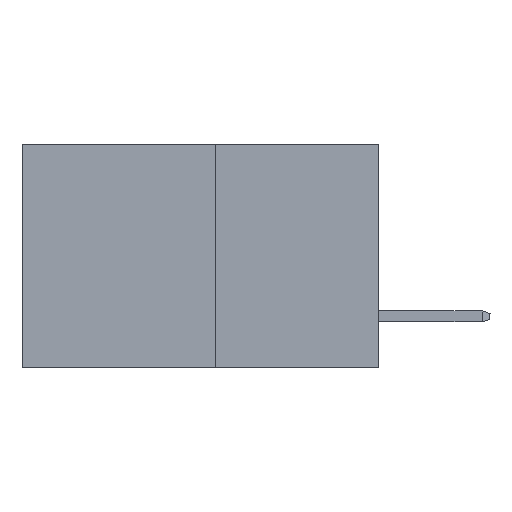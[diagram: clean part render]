
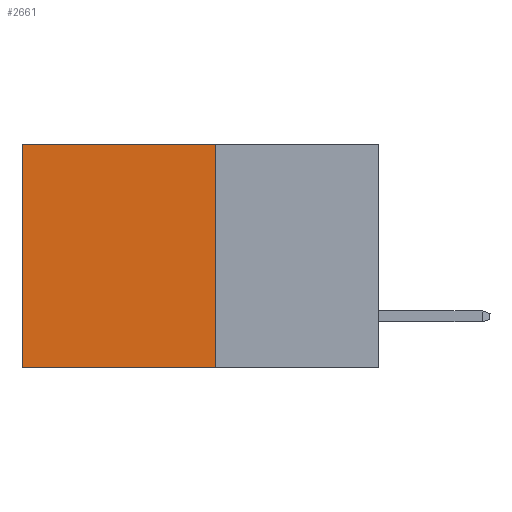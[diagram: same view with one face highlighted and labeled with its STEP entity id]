
A CAD part, left-side view. The second image highlights one B-rep face of the part: STEP entity #2661.
In plain terms, the highlighted planar face has unit normal (-1, 0, 0).
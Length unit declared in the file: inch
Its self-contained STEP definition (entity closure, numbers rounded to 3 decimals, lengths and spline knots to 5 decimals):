
#350 = LINE ( 'NONE', #3669, #9872 ) ;
#476 = EDGE_CURVE ( 'NONE', #3272, #10678, #350, .T. ) ;
#968 = EDGE_CURVE ( 'NONE', #11076, #4320, #6662, .T. ) ;
#1691 = VECTOR ( 'NONE', #6473, 39.37008 ) ;
#2283 = ORIENTED_EDGE ( 'NONE', *, *, #9791, .T. ) ;
#2437 = VECTOR ( 'NONE', #11187, 39.37008 ) ;
#2661 = ADVANCED_FACE ( 'NONE', ( #9771 ), #7723, .F. ) ;
#2718 = VECTOR ( 'NONE', #4957, 39.37008 ) ;
#2985 = AXIS2_PLACEMENT_3D ( 'NONE', #6815, #7709, #9764 ) ;
#3272 = VERTEX_POINT ( 'NONE', #7632 ) ;
#3622 = CARTESIAN_POINT ( 'NONE',  ( 0.277, 0.59, -0.37 ) ) ;
#3669 = CARTESIAN_POINT ( 'NONE',  ( 0.277, 0.27, 0. ) ) ;
#4080 = CARTESIAN_POINT ( 'NONE',  ( 0.277, 0.59, -0.37 ) ) ;
#4294 = LINE ( 'NONE', #4080, #2718 ) ;
#4320 = VERTEX_POINT ( 'NONE', #3622 ) ;
#4935 = ORIENTED_EDGE ( 'NONE', *, *, #6003, .F. ) ;
#4957 = DIRECTION ( 'NONE',  ( 0., 0., -1. ) ) ;
#5094 = EDGE_LOOP ( 'NONE', ( #2283, #5177, #4935, #7029 ) ) ;
#5177 = ORIENTED_EDGE ( 'NONE', *, *, #968, .F. ) ;
#5209 = CARTESIAN_POINT ( 'NONE',  ( 0.277, 0.27, -0.37 ) ) ;
#5261 = CARTESIAN_POINT ( 'NONE',  ( 0.277, 0.59, 0. ) ) ;
#5710 = CARTESIAN_POINT ( 'NONE',  ( 0.277, 0.27, -0.37 ) ) ;
#6003 = EDGE_CURVE ( 'NONE', #3272, #11076, #8776, .T. ) ;
#6473 = DIRECTION ( 'NONE',  ( 0., 0., -1. ) ) ;
#6662 = LINE ( 'NONE', #7329, #2437 ) ;
#6815 = CARTESIAN_POINT ( 'NONE',  ( 0.277, 0.27, -0.37 ) ) ;
#7029 = ORIENTED_EDGE ( 'NONE', *, *, #476, .T. ) ;
#7329 = CARTESIAN_POINT ( 'NONE',  ( 0.277, 0.27, -0.37 ) ) ;
#7632 = CARTESIAN_POINT ( 'NONE',  ( 0.277, 0.27, 0. ) ) ;
#7709 = DIRECTION ( 'NONE',  ( 1., 0., 0. ) ) ;
#7723 = PLANE ( 'NONE',  #2985 ) ;
#8718 = DIRECTION ( 'NONE',  ( 0., 1., 0. ) ) ;
#8776 = LINE ( 'NONE', #5209, #1691 ) ;
#9764 = DIRECTION ( 'NONE',  ( 0., 0., -1. ) ) ;
#9771 = FACE_OUTER_BOUND ( 'NONE', #5094, .T. ) ;
#9791 = EDGE_CURVE ( 'NONE', #10678, #4320, #4294, .T. ) ;
#9872 = VECTOR ( 'NONE', #8718, 39.37008 ) ;
#10678 = VERTEX_POINT ( 'NONE', #5261 ) ;
#11076 = VERTEX_POINT ( 'NONE', #5710 ) ;
#11187 = DIRECTION ( 'NONE',  ( 0., 1., 0. ) ) ;
